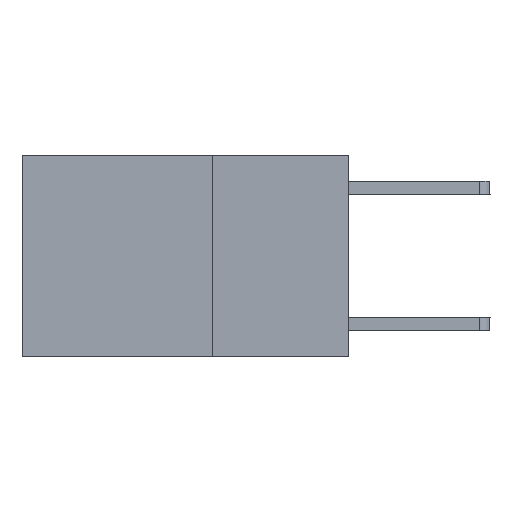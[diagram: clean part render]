
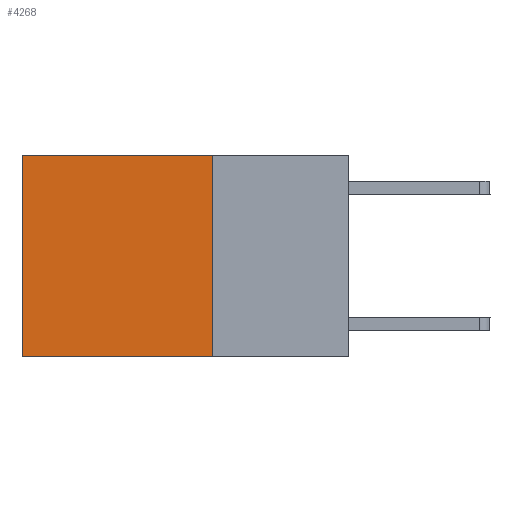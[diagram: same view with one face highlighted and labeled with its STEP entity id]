
A CAD part, left-side view. The second image highlights one B-rep face of the part: STEP entity #4268.
In plain terms, the highlighted planar face has unit normal (-1, 0, 0).
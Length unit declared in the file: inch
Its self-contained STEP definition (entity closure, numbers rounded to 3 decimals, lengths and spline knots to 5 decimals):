
#939 = DIRECTION ( 'NONE',  ( 0., 1., 0. ) ) ;
#1141 = EDGE_CURVE ( 'NONE', #8927, #5784, #8325, .T. ) ;
#1177 = DIRECTION ( 'NONE',  ( 0., 0., -1. ) ) ;
#2097 = CARTESIAN_POINT ( 'NONE',  ( 0.2625, 0.25, -0.37 ) ) ;
#2402 = CARTESIAN_POINT ( 'NONE',  ( 0.2625, 0.25, 0. ) ) ;
#3223 = DIRECTION ( 'NONE',  ( 0., 1., 0. ) ) ;
#3313 = DIRECTION ( 'NONE',  ( 0., 0., -1. ) ) ;
#3484 = LINE ( 'NONE', #10703, #3995 ) ;
#3712 = CARTESIAN_POINT ( 'NONE',  ( 0.2625, 0.25, -0.37 ) ) ;
#3970 = LINE ( 'NONE', #5808, #6097 ) ;
#3995 = VECTOR ( 'NONE', #4251, 39.37008 ) ;
#4251 = DIRECTION ( 'NONE',  ( 0., 0., -1. ) ) ;
#4268 = ADVANCED_FACE ( 'NONE', ( #11081 ), #11141, .F. ) ;
#4285 = ORIENTED_EDGE ( 'NONE', *, *, #1141, .F. ) ;
#4345 = LINE ( 'NONE', #2402, #11512 ) ;
#4690 = AXIS2_PLACEMENT_3D ( 'NONE', #5683, #10266, #1177 ) ;
#4799 = ORIENTED_EDGE ( 'NONE', *, *, #9782, .T. ) ;
#5683 = CARTESIAN_POINT ( 'NONE',  ( 0.2625, 0.25, 0. ) ) ;
#5784 = VERTEX_POINT ( 'NONE', #10539 ) ;
#5808 = CARTESIAN_POINT ( 'NONE',  ( 0.2625, 0.6, 0. ) ) ;
#5852 = VECTOR ( 'NONE', #939, 39.37008 ) ;
#5928 = CARTESIAN_POINT ( 'NONE',  ( 0.2625, 0.25, 0. ) ) ;
#6097 = VECTOR ( 'NONE', #3313, 39.37008 ) ;
#6362 = EDGE_CURVE ( 'NONE', #9364, #8927, #3484, .T. ) ;
#6677 = VERTEX_POINT ( 'NONE', #9709 ) ;
#7678 = ORIENTED_EDGE ( 'NONE', *, *, #8691, .T. ) ;
#8325 = LINE ( 'NONE', #3712, #5852 ) ;
#8691 = EDGE_CURVE ( 'NONE', #9364, #6677, #4345, .T. ) ;
#8927 = VERTEX_POINT ( 'NONE', #2097 ) ;
#9012 = EDGE_LOOP ( 'NONE', ( #4799, #4285, #10031, #7678 ) ) ;
#9364 = VERTEX_POINT ( 'NONE', #5928 ) ;
#9709 = CARTESIAN_POINT ( 'NONE',  ( 0.2625, 0.6, 0. ) ) ;
#9782 = EDGE_CURVE ( 'NONE', #6677, #5784, #3970, .T. ) ;
#10031 = ORIENTED_EDGE ( 'NONE', *, *, #6362, .F. ) ;
#10266 = DIRECTION ( 'NONE',  ( 1., 0., 0. ) ) ;
#10539 = CARTESIAN_POINT ( 'NONE',  ( 0.2625, 0.6, -0.37 ) ) ;
#10703 = CARTESIAN_POINT ( 'NONE',  ( 0.2625, 0.25, 0. ) ) ;
#11081 = FACE_OUTER_BOUND ( 'NONE', #9012, .T. ) ;
#11141 = PLANE ( 'NONE',  #4690 ) ;
#11512 = VECTOR ( 'NONE', #3223, 39.37008 ) ;
